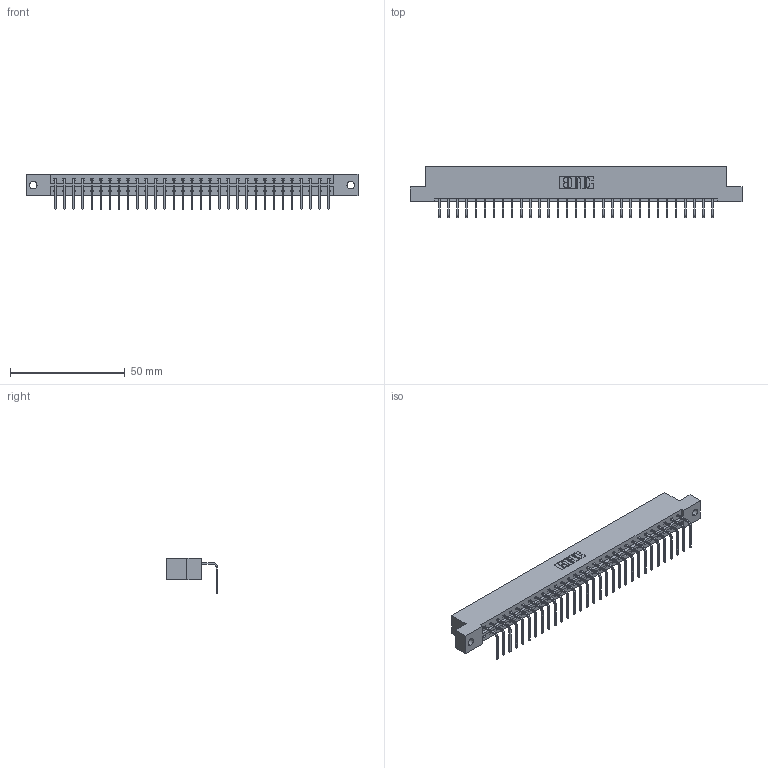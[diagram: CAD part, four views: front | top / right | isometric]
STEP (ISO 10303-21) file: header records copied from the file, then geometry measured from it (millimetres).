
FILE_DESCRIPTION (( 'STEP AP203' ), '1' );
FILE_NAME ('833-031-558-102.STEP', '2020-06-02T15:59:01', ( '' ), ( '' ), 'SwSTEP 2.0', 'SolidWorks 2020', '' );
FILE_SCHEMA (( 'CONFIG_CONTROL_DESIGN' ));
Length unit declared in the file: inch
Products named in the file (3): 833-031-558-102; 833 Part_Flush - .128 Dia; 345-292-001_558 Tail - 2
Assembly tree (32 placements, depth 2):
  833-031-558-102
    833 Part_Flush - .128 Dia
    345-292-001_558 Tail - 2  x31
Bounding box: 144.37 x 22.17 x 15.37 mm (x, y, z)
Volume: 14500.1 mm3; surface area: 15977.9 mm2
Topology: 32 solids, 32 shells, 1974 faces, 5953 edges, 3926 vertices
Faces by surface type: plane 1434, cylinder 540
Entity records: 20461 total; most frequent: CARTESIAN_POINT 3539, ORIENTED_EDGE 3506, DIRECTION 3007, EDGE_CURVE 1753, VECTOR 1625, LINE 1625, VERTEX_POINT 1166, AXIS2_PLACEMENT_3D 691
